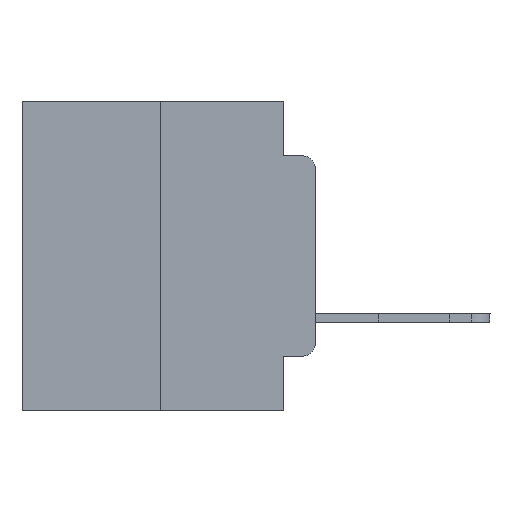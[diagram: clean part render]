
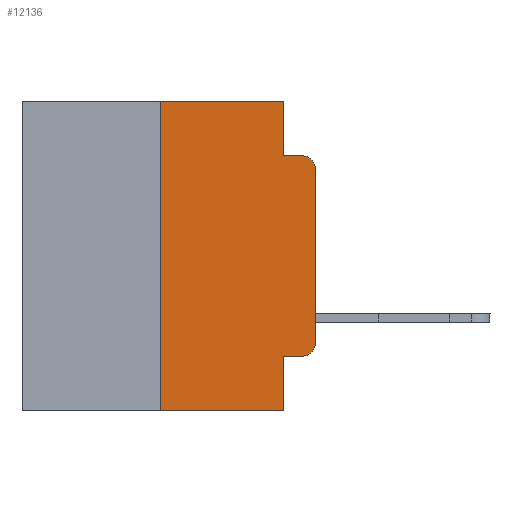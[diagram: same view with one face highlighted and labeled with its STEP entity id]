
A CAD part, left-side view. The second image highlights one B-rep face of the part: STEP entity #12136.
In plain terms, the highlighted planar face has unit normal (-1, 0, 0).
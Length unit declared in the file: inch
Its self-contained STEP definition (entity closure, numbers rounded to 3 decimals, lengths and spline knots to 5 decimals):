
#291 = CIRCLE ( 'NONE', #3598, 0.02 ) ;
#431 = EDGE_CURVE ( 'NONE', #10289, #11286, #291, .T. ) ;
#721 = ORIENTED_EDGE ( 'NONE', *, *, #9016, .T. ) ;
#949 = PLANE ( 'NONE',  #9511 ) ;
#956 = DIRECTION ( 'NONE',  ( 0., -1., 0. ) ) ;
#1309 = VERTEX_POINT ( 'NONE', #7778 ) ;
#1367 = ORIENTED_EDGE ( 'NONE', *, *, #5494, .F. ) ;
#1450 = DIRECTION ( 'NONE',  ( 0., 0., -1. ) ) ;
#1556 = CARTESIAN_POINT ( 'NONE',  ( 0., 0., 0. ) ) ;
#3274 = LINE ( 'NONE', #7159, #9971 ) ;
#3498 = VERTEX_POINT ( 'NONE', #9281 ) ;
#3598 = AXIS2_PLACEMENT_3D ( 'NONE', #19983, #19856, #14520 ) ;
#4196 = EDGE_CURVE ( 'NONE', #5306, #3498, #14823, .T. ) ;
#4513 = VECTOR ( 'NONE', #11555, 39.37008 ) ;
#5033 = CARTESIAN_POINT ( 'NONE',  ( 0., 0.02, -0.4115 ) ) ;
#5210 = DIRECTION ( 'NONE',  ( 0., -1., 0. ) ) ;
#5288 = VERTEX_POINT ( 'NONE', #22428 ) ;
#5306 = VERTEX_POINT ( 'NONE', #14491 ) ;
#5494 = EDGE_CURVE ( 'NONE', #1309, #21706, #19158, .T. ) ;
#5495 = LINE ( 'NONE', #9398, #8463 ) ;
#5527 = EDGE_CURVE ( 'NONE', #19360, #5306, #19276, .T. ) ;
#6651 = CARTESIAN_POINT ( 'NONE',  ( 0., 0.473, 0. ) ) ;
#7159 = CARTESIAN_POINT ( 'NONE',  ( 0., 0.473, -0.5 ) ) ;
#7737 = CARTESIAN_POINT ( 'NONE',  ( 0., 0., -0.3915 ) ) ;
#7778 = CARTESIAN_POINT ( 'NONE',  ( 0., 0.051, -0.4115 ) ) ;
#8463 = VECTOR ( 'NONE', #956, 39.37008 ) ;
#8515 = CARTESIAN_POINT ( 'NONE',  ( 0., 0., -0.1085 ) ) ;
#8760 = ORIENTED_EDGE ( 'NONE', *, *, #24646, .F. ) ;
#8968 = DIRECTION ( 'NONE',  ( 0., -1., 0. ) ) ;
#9016 = EDGE_CURVE ( 'NONE', #19360, #21706, #3274, .T. ) ;
#9230 = ORIENTED_EDGE ( 'NONE', *, *, #21081, .T. ) ;
#9281 = CARTESIAN_POINT ( 'NONE',  ( 0., 0.051, 0. ) ) ;
#9392 = CARTESIAN_POINT ( 'NONE',  ( 0., 0.25, 0. ) ) ;
#9398 = CARTESIAN_POINT ( 'NONE',  ( 0., 0.051, -0.0885 ) ) ;
#9511 = AXIS2_PLACEMENT_3D ( 'NONE', #16803, #22924, #14859 ) ;
#9614 = CARTESIAN_POINT ( 'NONE',  ( 0., 0.051, -0.5 ) ) ;
#9971 = VECTOR ( 'NONE', #5210, 39.37008 ) ;
#10010 = VERTEX_POINT ( 'NONE', #5033 ) ;
#10289 = VERTEX_POINT ( 'NONE', #8515 ) ;
#10669 = ORIENTED_EDGE ( 'NONE', *, *, #25674, .T. ) ;
#11286 = VERTEX_POINT ( 'NONE', #16664 ) ;
#11352 = EDGE_CURVE ( 'NONE', #1309, #10010, #19756, .T. ) ;
#11555 = DIRECTION ( 'NONE',  ( 0., 0., 1. ) ) ;
#11932 = VECTOR ( 'NONE', #1450, 39.37008 ) ;
#12136 = ADVANCED_FACE ( 'NONE', ( #16946 ), #949, .F. ) ;
#12263 = VECTOR ( 'NONE', #15470, 39.37008 ) ;
#12500 = ORIENTED_EDGE ( 'NONE', *, *, #4196, .F. ) ;
#12660 = CARTESIAN_POINT ( 'NONE',  ( 0., 0.051, 0. ) ) ;
#13230 = VECTOR ( 'NONE', #13559, 39.37008 ) ;
#13395 = CARTESIAN_POINT ( 'NONE',  ( 0., 0.051, -0.4115 ) ) ;
#13435 = CIRCLE ( 'NONE', #15513, 0.02 ) ;
#13501 = LINE ( 'NONE', #1556, #4513 ) ;
#13559 = DIRECTION ( 'NONE',  ( 0., 0., 1. ) ) ;
#13576 = VECTOR ( 'NONE', #8968, 39.37008 ) ;
#14352 = DIRECTION ( 'NONE',  ( -1., 0., 0. ) ) ;
#14491 = CARTESIAN_POINT ( 'NONE',  ( 0., 0.25, 0. ) ) ;
#14520 = DIRECTION ( 'NONE',  ( 0., 0., -1. ) ) ;
#14823 = LINE ( 'NONE', #6651, #13576 ) ;
#14859 = DIRECTION ( 'NONE',  ( 0., 0., -1. ) ) ;
#14866 = VECTOR ( 'NONE', #20594, 39.37008 ) ;
#15221 = CARTESIAN_POINT ( 'NONE',  ( 0., 0.051, 0. ) ) ;
#15359 = LINE ( 'NONE', #15221, #11932 ) ;
#15470 = DIRECTION ( 'NONE',  ( 0., -1., 0. ) ) ;
#15513 = AXIS2_PLACEMENT_3D ( 'NONE', #16436, #14352, #24244 ) ;
#15642 = ORIENTED_EDGE ( 'NONE', *, *, #5527, .F. ) ;
#15987 = EDGE_CURVE ( 'NONE', #5288, #11286, #5495, .T. ) ;
#16436 = CARTESIAN_POINT ( 'NONE',  ( 0., 0.02, -0.3915 ) ) ;
#16664 = CARTESIAN_POINT ( 'NONE',  ( 0., 0.02, -0.0885 ) ) ;
#16803 = CARTESIAN_POINT ( 'NONE',  ( 0., 0.473, 0. ) ) ;
#16946 = FACE_OUTER_BOUND ( 'NONE', #21824, .T. ) ;
#17057 = VERTEX_POINT ( 'NONE', #7737 ) ;
#19158 = LINE ( 'NONE', #12660, #14866 ) ;
#19276 = LINE ( 'NONE', #9392, #13230 ) ;
#19360 = VERTEX_POINT ( 'NONE', #24024 ) ;
#19690 = ORIENTED_EDGE ( 'NONE', *, *, #11352, .T. ) ;
#19756 = LINE ( 'NONE', #13395, #12263 ) ;
#19856 = DIRECTION ( 'NONE',  ( -1., 0., 0. ) ) ;
#19983 = CARTESIAN_POINT ( 'NONE',  ( 0., 0.02, -0.1085 ) ) ;
#20594 = DIRECTION ( 'NONE',  ( 0., 0., -1. ) ) ;
#21081 = EDGE_CURVE ( 'NONE', #10010, #17057, #13435, .T. ) ;
#21440 = ORIENTED_EDGE ( 'NONE', *, *, #431, .T. ) ;
#21706 = VERTEX_POINT ( 'NONE', #9614 ) ;
#21824 = EDGE_LOOP ( 'NONE', ( #10669, #21440, #24976, #8760, #12500, #15642, #721, #1367, #19690, #9230 ) ) ;
#22428 = CARTESIAN_POINT ( 'NONE',  ( 0., 0.051, -0.0885 ) ) ;
#22924 = DIRECTION ( 'NONE',  ( 1., 0., 0. ) ) ;
#24024 = CARTESIAN_POINT ( 'NONE',  ( 0., 0.25, -0.5 ) ) ;
#24244 = DIRECTION ( 'NONE',  ( 0., 0., -1. ) ) ;
#24646 = EDGE_CURVE ( 'NONE', #3498, #5288, #15359, .T. ) ;
#24976 = ORIENTED_EDGE ( 'NONE', *, *, #15987, .F. ) ;
#25674 = EDGE_CURVE ( 'NONE', #17057, #10289, #13501, .T. ) ;
